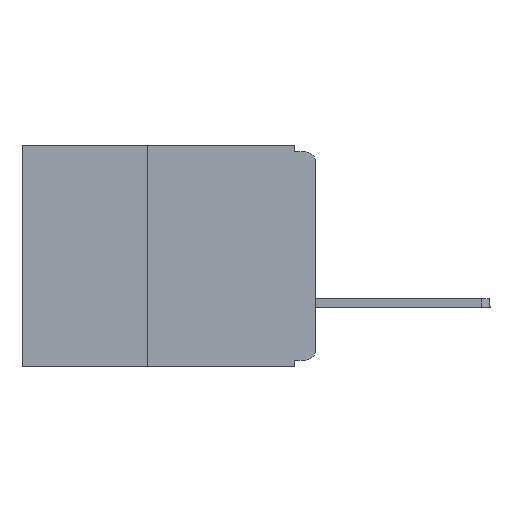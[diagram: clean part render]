
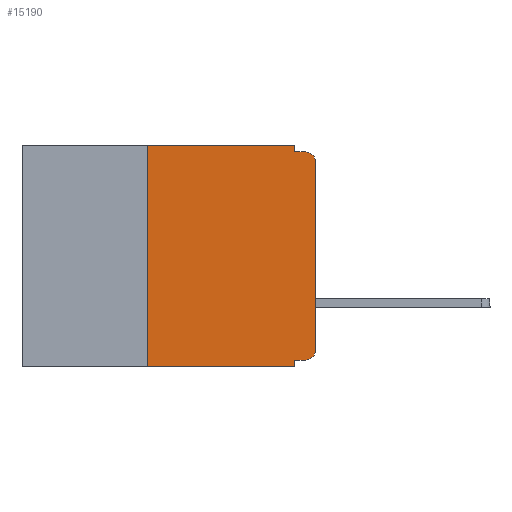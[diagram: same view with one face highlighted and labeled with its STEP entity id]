
A CAD part, left-side view. The second image highlights one B-rep face of the part: STEP entity #15190.
In plain terms, the highlighted planar face has unit normal (-1, 0, 0).
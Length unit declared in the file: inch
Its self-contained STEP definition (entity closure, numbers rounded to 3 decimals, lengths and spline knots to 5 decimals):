
#428 = DIRECTION ( 'NONE',  ( 0., 0., -1. ) ) ;
#459 = DIRECTION ( 'NONE',  ( -1., 0., 0. ) ) ;
#488 = CARTESIAN_POINT ( 'NONE',  ( 0., 0.015, -0.025 ) ) ;
#691 = FACE_OUTER_BOUND ( 'NONE', #4883, .T. ) ;
#1710 = VECTOR ( 'NONE', #3284, 39.37008 ) ;
#1782 = VECTOR ( 'NONE', #14018, 39.37008 ) ;
#2232 = VECTOR ( 'NONE', #9228, 39.37008 ) ;
#2503 = ORIENTED_EDGE ( 'NONE', *, *, #15347, .F. ) ;
#2714 = CARTESIAN_POINT ( 'NONE',  ( 0., 0.031, 0. ) ) ;
#3284 = DIRECTION ( 'NONE',  ( 0., 0., -1. ) ) ;
#3334 = CARTESIAN_POINT ( 'NONE',  ( 0., 0.031, -0.33 ) ) ;
#3833 = VERTEX_POINT ( 'NONE', #18309 ) ;
#3999 = LINE ( 'NONE', #16809, #19265 ) ;
#4203 = VERTEX_POINT ( 'NONE', #3334 ) ;
#4483 = VERTEX_POINT ( 'NONE', #20279 ) ;
#4727 = CARTESIAN_POINT ( 'NONE',  ( 0., 0.437, 0. ) ) ;
#4729 = LINE ( 'NONE', #5583, #10256 ) ;
#4883 = EDGE_LOOP ( 'NONE', ( #7042, #18462, #5775, #2503, #23317, #18522, #13355, #12732, #12409, #6513 ) ) ;
#5117 = DIRECTION ( 'NONE',  ( 0., -1., 0. ) ) ;
#5445 = VERTEX_POINT ( 'NONE', #18365 ) ;
#5497 = VECTOR ( 'NONE', #13161, 39.37008 ) ;
#5583 = CARTESIAN_POINT ( 'NONE',  ( 0., 0., -0.01 ) ) ;
#5718 = CARTESIAN_POINT ( 'NONE',  ( 0., 0., 0. ) ) ;
#5775 = ORIENTED_EDGE ( 'NONE', *, *, #14320, .F. ) ;
#6513 = ORIENTED_EDGE ( 'NONE', *, *, #25777, .T. ) ;
#6736 = CIRCLE ( 'NONE', #15447, 0.015 ) ;
#7042 = ORIENTED_EDGE ( 'NONE', *, *, #19416, .T. ) ;
#7856 = EDGE_CURVE ( 'NONE', #14953, #3833, #22766, .T. ) ;
#7936 = LINE ( 'NONE', #25718, #12820 ) ;
#8651 = CARTESIAN_POINT ( 'NONE',  ( 0., 0.25, 0. ) ) ;
#8828 = EDGE_CURVE ( 'NONE', #14165, #4203, #7936, .T. ) ;
#8848 = CARTESIAN_POINT ( 'NONE',  ( 0., 0.015, -0.32 ) ) ;
#9228 = DIRECTION ( 'NONE',  ( 0., -1., 0. ) ) ;
#9326 = DIRECTION ( 'NONE',  ( -1., 0., 0. ) ) ;
#9897 = EDGE_CURVE ( 'NONE', #20369, #14165, #3999, .T. ) ;
#10256 = VECTOR ( 'NONE', #22218, 39.37008 ) ;
#10639 = DIRECTION ( 'NONE',  ( 0., 1., 0. ) ) ;
#12003 = LINE ( 'NONE', #21654, #2232 ) ;
#12409 = ORIENTED_EDGE ( 'NONE', *, *, #9897, .F. ) ;
#12732 = ORIENTED_EDGE ( 'NONE', *, *, #8828, .F. ) ;
#12820 = VECTOR ( 'NONE', #15399, 39.37008 ) ;
#13099 = DIRECTION ( 'NONE',  ( 0., 0., -1. ) ) ;
#13161 = DIRECTION ( 'NONE',  ( 0., 0., 1. ) ) ;
#13355 = ORIENTED_EDGE ( 'NONE', *, *, #18929, .T. ) ;
#14018 = DIRECTION ( 'NONE',  ( 0., 0., 1. ) ) ;
#14165 = VERTEX_POINT ( 'NONE', #25795 ) ;
#14320 = EDGE_CURVE ( 'NONE', #21957, #3833, #4729, .T. ) ;
#14612 = AXIS2_PLACEMENT_3D ( 'NONE', #4727, #25476, #13099 ) ;
#14781 = VECTOR ( 'NONE', #5117, 39.37008 ) ;
#14953 = VERTEX_POINT ( 'NONE', #24711 ) ;
#15190 = ADVANCED_FACE ( 'NONE', ( #691 ), #23432, .F. ) ;
#15347 = EDGE_CURVE ( 'NONE', #18225, #21957, #18262, .T. ) ;
#15399 = DIRECTION ( 'NONE',  ( 0., 0., -1. ) ) ;
#15447 = AXIS2_PLACEMENT_3D ( 'NONE', #21762, #9326, #23844 ) ;
#16439 = EDGE_CURVE ( 'NONE', #5445, #26221, #16559, .T. ) ;
#16559 = LINE ( 'NONE', #25543, #5497 ) ;
#16809 = CARTESIAN_POINT ( 'NONE',  ( 0., 0., -0.32 ) ) ;
#17033 = EDGE_CURVE ( 'NONE', #26221, #18225, #12003, .T. ) ;
#17588 = AXIS2_PLACEMENT_3D ( 'NONE', #488, #459, #428 ) ;
#18225 = VERTEX_POINT ( 'NONE', #2714 ) ;
#18262 = LINE ( 'NONE', #23958, #1710 ) ;
#18309 = CARTESIAN_POINT ( 'NONE',  ( 0., 0.015, -0.01 ) ) ;
#18344 = LINE ( 'NONE', #5718, #1782 ) ;
#18365 = CARTESIAN_POINT ( 'NONE',  ( 0., 0.25, -0.33 ) ) ;
#18462 = ORIENTED_EDGE ( 'NONE', *, *, #7856, .T. ) ;
#18522 = ORIENTED_EDGE ( 'NONE', *, *, #16439, .F. ) ;
#18780 = CARTESIAN_POINT ( 'NONE',  ( 0., 0.031, -0.01 ) ) ;
#18929 = EDGE_CURVE ( 'NONE', #5445, #4203, #20323, .T. ) ;
#19265 = VECTOR ( 'NONE', #10639, 39.37008 ) ;
#19416 = EDGE_CURVE ( 'NONE', #4483, #14953, #18344, .T. ) ;
#20279 = CARTESIAN_POINT ( 'NONE',  ( 0., 0., -0.305 ) ) ;
#20323 = LINE ( 'NONE', #25782, #14781 ) ;
#20369 = VERTEX_POINT ( 'NONE', #8848 ) ;
#21654 = CARTESIAN_POINT ( 'NONE',  ( 0., 0.437, 0. ) ) ;
#21762 = CARTESIAN_POINT ( 'NONE',  ( 0., 0.015, -0.305 ) ) ;
#21957 = VERTEX_POINT ( 'NONE', #18780 ) ;
#22218 = DIRECTION ( 'NONE',  ( 0., -1., 0. ) ) ;
#22766 = CIRCLE ( 'NONE', #17588, 0.015 ) ;
#23317 = ORIENTED_EDGE ( 'NONE', *, *, #17033, .F. ) ;
#23432 = PLANE ( 'NONE',  #14612 ) ;
#23844 = DIRECTION ( 'NONE',  ( 0., 0., -1. ) ) ;
#23958 = CARTESIAN_POINT ( 'NONE',  ( 0., 0.031, 0. ) ) ;
#24711 = CARTESIAN_POINT ( 'NONE',  ( 0., 0., -0.025 ) ) ;
#25476 = DIRECTION ( 'NONE',  ( 1., 0., 0. ) ) ;
#25543 = CARTESIAN_POINT ( 'NONE',  ( 0., 0.25, -0.33 ) ) ;
#25718 = CARTESIAN_POINT ( 'NONE',  ( 0., 0.031, -0.33 ) ) ;
#25777 = EDGE_CURVE ( 'NONE', #20369, #4483, #6736, .T. ) ;
#25782 = CARTESIAN_POINT ( 'NONE',  ( 0., 0.437, -0.33 ) ) ;
#25795 = CARTESIAN_POINT ( 'NONE',  ( 0., 0.031, -0.32 ) ) ;
#26221 = VERTEX_POINT ( 'NONE', #8651 ) ;
